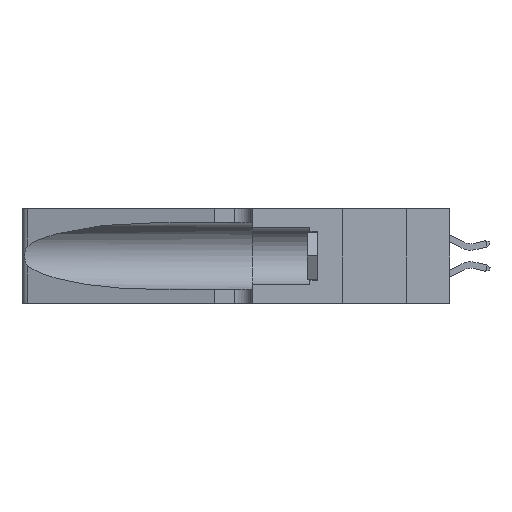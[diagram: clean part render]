
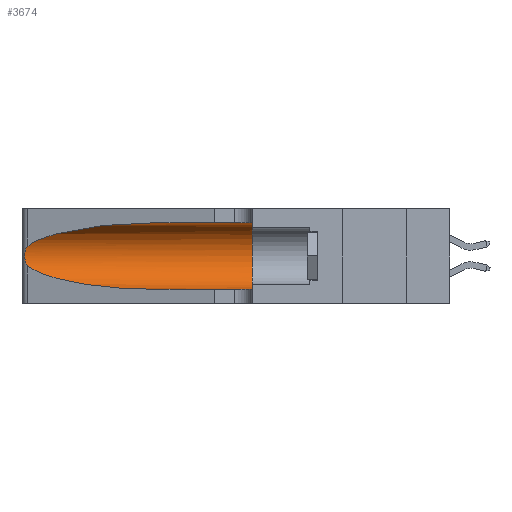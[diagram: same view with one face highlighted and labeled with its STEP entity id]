
A CAD part, left-side view. The second image highlights one B-rep face of the part: STEP entity #3674.
In plain terms, the highlighted cylindrical face has radius 3.308 mm (diameter 6.617 mm), a partial arc.
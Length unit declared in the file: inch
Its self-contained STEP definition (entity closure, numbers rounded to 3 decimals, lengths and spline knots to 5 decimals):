
#240 = CARTESIAN_POINT ( 'NONE',  ( 0.25487, 1.22718, 0.14631 ) ) ;
#466 = FACE_OUTER_BOUND ( 'NONE', #6168, .T. ) ;
#1185 = DIRECTION ( 'NONE',  ( 0., -1., 0. ) ) ;
#1249 = CARTESIAN_POINT ( 'NONE',  ( 0.26017, 1.23833, 0.17102 ) ) ;
#1254 = VECTOR ( 'NONE', #1185, 39.37008 ) ;
#1319 = VERTEX_POINT ( 'NONE', #10164 ) ;
#2308 = VECTOR ( 'NONE', #11340, 39.37008 ) ;
#2812 = CARTESIAN_POINT ( 'NONE',  ( 0.25789, 1.23486, 0.15765 ) ) ;
#2853 = CARTESIAN_POINT ( 'NONE',  ( 0.25487, 1.22718, 0.14631 ) ) ;
#3161 = B_SPLINE_CURVE_WITH_KNOTS ( 'NONE', 3,
 ( #14637, #4288, #16092, #7342, #17570, #8864, #19006, #10323, #1249, #11776, #2812, #13260, #4358, #14701 ),
 .UNSPECIFIED., .F., .F.,
 ( 4, 2, 2, 2, 2, 2, 4 ),
 ( 0., 0.00027, 0.00053, 0.00107, 0.0016, 0.00187, 0.00214 ),
 .UNSPECIFIED. ) ;
#3674 = ADVANCED_FACE ( 'NONE', ( #466 ), #11107, .F. ) ;
#3816 = CARTESIAN_POINT ( 'NONE',  ( 0.1305, 1.61858, 0.05475 ) ) ;
#4288 = CARTESIAN_POINT ( 'NONE',  ( 0.25555, 1.22994, 0.2215 ) ) ;
#4358 = CARTESIAN_POINT ( 'NONE',  ( 0.25555, 1.22993, 0.14849 ) ) ;
#4402 = CARTESIAN_POINT ( 'NONE',  ( 0.1305, 0.72297, 0.05475 ) ) ;
#4494 = CIRCLE ( 'NONE', #16320, 0.13025 ) ;
#4808 = ORIENTED_EDGE ( 'NONE', *, *, #11923, .T. ) ;
#4957 = DIRECTION ( 'NONE',  ( 0., 1., 0. ) ) ;
#5128 = CARTESIAN_POINT ( 'NONE',  ( 0.18966, 0.96281, 0.31525 ) ) ;
#5336 = ORIENTED_EDGE ( 'NONE', *, *, #18612, .F. ) ;
#5816 = LINE ( 'NONE', #16036, #1254 ) ;
#6168 = EDGE_LOOP ( 'NONE', ( #18527, #12340, #18119, #4808, #7474, #5336 ) ) ;
#6887 = VERTEX_POINT ( 'NONE', #10129 ) ;
#7005 = VERTEX_POINT ( 'NONE', #14763 ) ;
#7342 = CARTESIAN_POINT ( 'NONE',  ( 0.25787, 1.23484, 0.2124 ) ) ;
#7474 = ORIENTED_EDGE ( 'NONE', *, *, #16429, .F. ) ;
#7647 = EDGE_CURVE ( 'NONE', #15759, #12903, #10928, .T. ) ;
#8638 = DIRECTION ( 'NONE',  ( 0., -1., 0. ) ) ;
#8864 = CARTESIAN_POINT ( 'NONE',  ( 0.26018, 1.23835, 0.19895 ) ) ;
#9658 = CARTESIAN_POINT ( 'NONE',  ( 0.25487, 1.22718, 0.22369 ) ) ;
#10129 = CARTESIAN_POINT ( 'NONE',  ( 0.1305, 0.35, 0.31525 ) ) ;
#10164 = CARTESIAN_POINT ( 'NONE',  ( 0.1305, 0.35, 0.05475 ) ) ;
#10323 = CARTESIAN_POINT ( 'NONE',  ( 0.26075, 1.23896, 0.178 ) ) ;
#10928 =( BOUNDED_CURVE ( )  B_SPLINE_CURVE ( 3, ( #2853, #17609, #11817, #4402 ),
 .UNSPECIFIED., .F., .T. ) 
 B_SPLINE_CURVE_WITH_KNOTS ( ( 4, 4 ),
 ( 3.44316, 4.71239 ),
 .UNSPECIFIED. ) 
 CURVE ( )  GEOMETRIC_REPRESENTATION_ITEM ( )  RATIONAL_B_SPLINE_CURVE ( ( 1., 0.87, 0.87, 1. ) ) 
 REPRESENTATION_ITEM ( '' )  );
#11107 = CYLINDRICAL_SURFACE ( 'NONE', #18436, 0.13025 ) ;
#11340 = DIRECTION ( 'NONE',  ( 0., -1., 0. ) ) ;
#11776 = CARTESIAN_POINT ( 'NONE',  ( 0.25856, 1.23593, 0.16098 ) ) ;
#11817 = CARTESIAN_POINT ( 'NONE',  ( 0.18966, 0.96281, 0.05475 ) ) ;
#11923 = EDGE_CURVE ( 'NONE', #12903, #1319, #14198, .T. ) ;
#12121 =( BOUNDED_CURVE ( )  B_SPLINE_CURVE ( 3, ( #13915, #5128, #18357, #9658 ),
 .UNSPECIFIED., .F., .T. ) 
 B_SPLINE_CURVE_WITH_KNOTS ( ( 4, 4 ),
 ( 1.5708, 2.84003 ),
 .UNSPECIFIED. ) 
 CURVE ( )  GEOMETRIC_REPRESENTATION_ITEM ( )  RATIONAL_B_SPLINE_CURVE ( ( 1., 0.87, 0.87, 1. ) ) 
 REPRESENTATION_ITEM ( '' )  );
#12340 = ORIENTED_EDGE ( 'NONE', *, *, #14354, .T. ) ;
#12744 = VERTEX_POINT ( 'NONE', #17354 ) ;
#12903 = VERTEX_POINT ( 'NONE', #14880 ) ;
#13260 = CARTESIAN_POINT ( 'NONE',  ( 0.25639, 1.23186, 0.15144 ) ) ;
#13804 = CARTESIAN_POINT ( 'NONE',  ( 0.1305, 0.35, 0.185 ) ) ;
#13915 = CARTESIAN_POINT ( 'NONE',  ( 0.1305, 0.72297, 0.31525 ) ) ;
#14198 = LINE ( 'NONE', #3816, #2308 ) ;
#14354 = EDGE_CURVE ( 'NONE', #7005, #15759, #3161, .T. ) ;
#14423 = DIRECTION ( 'NONE',  ( 0., 0., -1. ) ) ;
#14637 = CARTESIAN_POINT ( 'NONE',  ( 0.25487, 1.22718, 0.22369 ) ) ;
#14701 = CARTESIAN_POINT ( 'NONE',  ( 0.25487, 1.22718, 0.14631 ) ) ;
#14763 = CARTESIAN_POINT ( 'NONE',  ( 0.25487, 1.22718, 0.22369 ) ) ;
#14880 = CARTESIAN_POINT ( 'NONE',  ( 0.1305, 0.72297, 0.05475 ) ) ;
#15181 = EDGE_CURVE ( 'NONE', #12744, #7005, #12121, .T. ) ;
#15243 = DIRECTION ( 'NONE',  ( 0., 0., 1. ) ) ;
#15759 = VERTEX_POINT ( 'NONE', #240 ) ;
#16036 = CARTESIAN_POINT ( 'NONE',  ( 0.1305, 1.61858, 0.31525 ) ) ;
#16092 = CARTESIAN_POINT ( 'NONE',  ( 0.25639, 1.23184, 0.21858 ) ) ;
#16320 = AXIS2_PLACEMENT_3D ( 'NONE', #13804, #4957, #15243 ) ;
#16429 = EDGE_CURVE ( 'NONE', #6887, #1319, #4494, .T. ) ;
#17354 = CARTESIAN_POINT ( 'NONE',  ( 0.1305, 0.72297, 0.31525 ) ) ;
#17570 = CARTESIAN_POINT ( 'NONE',  ( 0.25854, 1.2359, 0.20912 ) ) ;
#17609 = CARTESIAN_POINT ( 'NONE',  ( 0.2373, 1.15595, 0.08982 ) ) ;
#18119 = ORIENTED_EDGE ( 'NONE', *, *, #7647, .T. ) ;
#18357 = CARTESIAN_POINT ( 'NONE',  ( 0.2373, 1.15595, 0.28018 ) ) ;
#18436 = AXIS2_PLACEMENT_3D ( 'NONE', #18787, #8638, #14423 ) ;
#18527 = ORIENTED_EDGE ( 'NONE', *, *, #15181, .T. ) ;
#18612 = EDGE_CURVE ( 'NONE', #12744, #6887, #5816, .T. ) ;
#18787 = CARTESIAN_POINT ( 'NONE',  ( 0.1305, 1.61858, 0.185 ) ) ;
#19006 = CARTESIAN_POINT ( 'NONE',  ( 0.26075, 1.23896, 0.19203 ) ) ;
